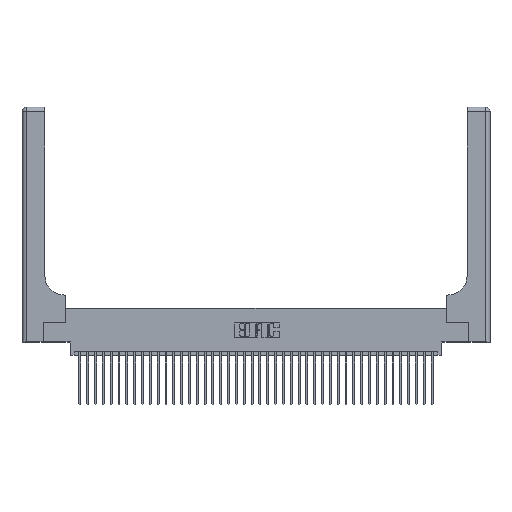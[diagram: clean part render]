
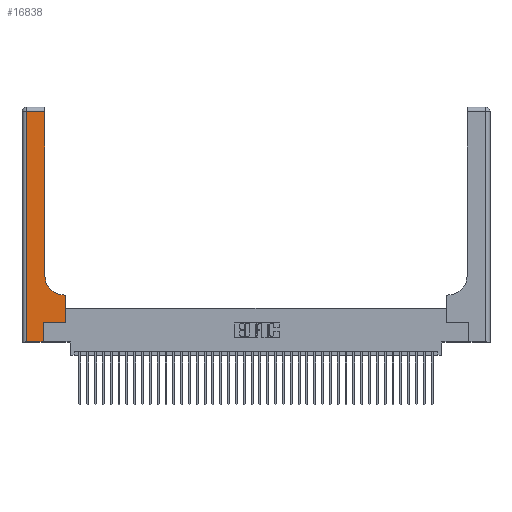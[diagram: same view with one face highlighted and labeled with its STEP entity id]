
A CAD part, top view. The second image highlights one B-rep face of the part: STEP entity #16838.
In plain terms, the highlighted planar face has unit normal (0, 0, 1).
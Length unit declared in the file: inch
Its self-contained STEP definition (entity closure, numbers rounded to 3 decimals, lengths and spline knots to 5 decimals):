
#712 = CARTESIAN_POINT ( 'NONE',  ( 0.269, 0., 0.37 ) ) ;
#1122 = LINE ( 'NONE', #25670, #10483 ) ;
#1241 = VECTOR ( 'NONE', #6666, 39.37008 ) ;
#2246 = VERTEX_POINT ( 'NONE', #12784 ) ;
#3021 = ORIENTED_EDGE ( 'NONE', *, *, #35941, .T. ) ;
#3485 = DIRECTION ( 'NONE',  ( 0., 1., 0. ) ) ;
#3995 = DIRECTION ( 'NONE',  ( -1., 0., 0. ) ) ;
#6666 = DIRECTION ( 'NONE',  ( 0., 1., 0. ) ) ;
#6779 = CARTESIAN_POINT ( 'NONE',  ( 0.2915, 3., 0.37 ) ) ;
#7788 = CARTESIAN_POINT ( 'NONE',  ( 0.5415, 0.6, 0.37 ) ) ;
#7828 = VERTEX_POINT ( 'NONE', #25255 ) ;
#8451 = ORIENTED_EDGE ( 'NONE', *, *, #14672, .T. ) ;
#8452 = DIRECTION ( 'NONE',  ( 0., 0., -1. ) ) ;
#8940 = ORIENTED_EDGE ( 'NONE', *, *, #38934, .T. ) ;
#9301 = VECTOR ( 'NONE', #3485, 39.37008 ) ;
#9391 = VERTEX_POINT ( 'NONE', #10183 ) ;
#9540 = DIRECTION ( 'NONE',  ( 1., 0., 0. ) ) ;
#9609 = VECTOR ( 'NONE', #12337, 39.37008 ) ;
#10183 = CARTESIAN_POINT ( 'NONE',  ( 0.2915, 2.94, 0.37 ) ) ;
#10483 = VECTOR ( 'NONE', #35263, 39.37008 ) ;
#10938 = AXIS2_PLACEMENT_3D ( 'NONE', #14934, #8452, #11909 ) ;
#11083 = LINE ( 'NONE', #34971, #1241 ) ;
#11162 = VECTOR ( 'NONE', #21705, 39.37008 ) ;
#11436 = VECTOR ( 'NONE', #21032, 39.37008 ) ;
#11845 = FACE_OUTER_BOUND ( 'NONE', #39598, .T. ) ;
#11909 = DIRECTION ( 'NONE',  ( -1., 0., 0. ) ) ;
#12272 = CIRCLE ( 'NONE', #37045, 0.25 ) ;
#12337 = DIRECTION ( 'NONE',  ( 1., 0., 0. ) ) ;
#12698 = DIRECTION ( 'NONE',  ( 0., 0., -1. ) ) ;
#12784 = CARTESIAN_POINT ( 'NONE',  ( 0.5585, 0.6, 0.37 ) ) ;
#13017 = VECTOR ( 'NONE', #36325, 39.37008 ) ;
#14452 = EDGE_CURVE ( 'NONE', #9391, #37459, #40252, .T. ) ;
#14470 = ORIENTED_EDGE ( 'NONE', *, *, #14452, .T. ) ;
#14672 = EDGE_CURVE ( 'NONE', #2246, #29246, #38793, .T. ) ;
#14934 = CARTESIAN_POINT ( 'NONE',  ( 0., 3., 0.37 ) ) ;
#15231 = VERTEX_POINT ( 'NONE', #22024 ) ;
#15916 = ORIENTED_EDGE ( 'NONE', *, *, #29465, .T. ) ;
#16838 = ADVANCED_FACE ( 'NONE', ( #11845 ), #34000, .F. ) ;
#17850 = CARTESIAN_POINT ( 'NONE',  ( 0., 0., 0.37 ) ) ;
#19186 = LINE ( 'NONE', #6779, #9301 ) ;
#20013 = LINE ( 'NONE', #27805, #9609 ) ;
#20825 = ORIENTED_EDGE ( 'NONE', *, *, #33568, .T. ) ;
#21032 = DIRECTION ( 'NONE',  ( 1., 0., 0. ) ) ;
#21705 = DIRECTION ( 'NONE',  ( 0., -1., 0. ) ) ;
#22024 = CARTESIAN_POINT ( 'NONE',  ( 0.269, 0.25, 0.37 ) ) ;
#22529 = LINE ( 'NONE', #30350, #11162 ) ;
#22562 = ORIENTED_EDGE ( 'NONE', *, *, #27497, .T. ) ;
#23774 = LINE ( 'NONE', #17850, #11436 ) ;
#24247 = VERTEX_POINT ( 'NONE', #712 ) ;
#24508 = VERTEX_POINT ( 'NONE', #24720 ) ;
#24720 = CARTESIAN_POINT ( 'NONE',  ( 0.2915, 0.85, 0.37 ) ) ;
#25255 = CARTESIAN_POINT ( 'NONE',  ( 0.5585, 0.25, 0.37 ) ) ;
#25256 = CARTESIAN_POINT ( 'NONE',  ( 0.5415, 0.85, 0.37 ) ) ;
#25602 = CARTESIAN_POINT ( 'NONE',  ( 0., 2.94, 0.37 ) ) ;
#25670 = CARTESIAN_POINT ( 'NONE',  ( 0.269, 0., 0.37 ) ) ;
#27497 = EDGE_CURVE ( 'NONE', #15231, #7828, #20013, .T. ) ;
#27805 = CARTESIAN_POINT ( 'NONE',  ( 0.269, 0.25, 0.37 ) ) ;
#28535 = ORIENTED_EDGE ( 'NONE', *, *, #37858, .T. ) ;
#29246 = VERTEX_POINT ( 'NONE', #7788 ) ;
#29465 = EDGE_CURVE ( 'NONE', #36812, #24247, #23774, .T. ) ;
#29896 = CARTESIAN_POINT ( 'NONE',  ( 0.2915, 0.6, 0.37 ) ) ;
#30350 = CARTESIAN_POINT ( 'NONE',  ( 0.06, 3., 0.37 ) ) ;
#31797 = VECTOR ( 'NONE', #3995, 39.37008 ) ;
#33387 = EDGE_CURVE ( 'NONE', #29246, #24508, #12272, .T. ) ;
#33568 = EDGE_CURVE ( 'NONE', #24508, #9391, #19186, .T. ) ;
#34000 = PLANE ( 'NONE',  #10938 ) ;
#34971 = CARTESIAN_POINT ( 'NONE',  ( 0.5585, 0.25, 0.37 ) ) ;
#35263 = DIRECTION ( 'NONE',  ( 0., 1., 0. ) ) ;
#35941 = EDGE_CURVE ( 'NONE', #7828, #2246, #11083, .T. ) ;
#36325 = DIRECTION ( 'NONE',  ( -1., 0., 0. ) ) ;
#36812 = VERTEX_POINT ( 'NONE', #36889 ) ;
#36889 = CARTESIAN_POINT ( 'NONE',  ( 0.06, 0., 0.37 ) ) ;
#37045 = AXIS2_PLACEMENT_3D ( 'NONE', #25256, #12698, #9540 ) ;
#37459 = VERTEX_POINT ( 'NONE', #40003 ) ;
#37858 = EDGE_CURVE ( 'NONE', #24247, #15231, #1122, .T. ) ;
#38793 = LINE ( 'NONE', #29896, #13017 ) ;
#38934 = EDGE_CURVE ( 'NONE', #37459, #36812, #22529, .T. ) ;
#39291 = ORIENTED_EDGE ( 'NONE', *, *, #33387, .T. ) ;
#39598 = EDGE_LOOP ( 'NONE', ( #20825, #14470, #8940, #15916, #28535, #22562, #3021, #8451, #39291 ) ) ;
#40003 = CARTESIAN_POINT ( 'NONE',  ( 0.06, 2.94, 0.37 ) ) ;
#40252 = LINE ( 'NONE', #25602, #31797 ) ;
